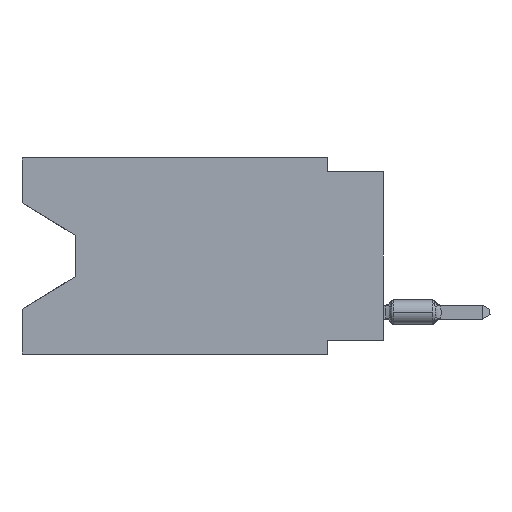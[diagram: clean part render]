
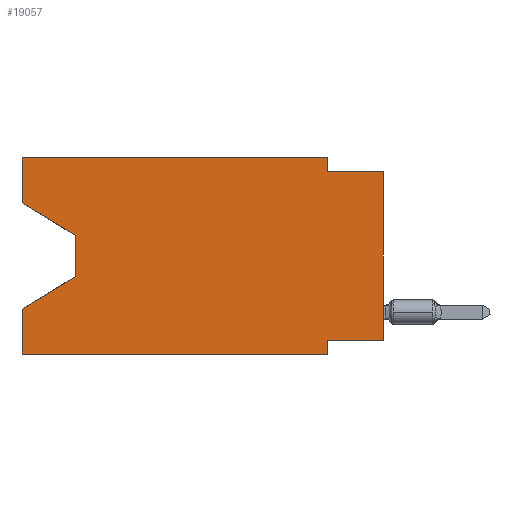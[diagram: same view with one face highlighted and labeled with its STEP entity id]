
A CAD part, left-side view. The second image highlights one B-rep face of the part: STEP entity #19057.
In plain terms, the highlighted planar face has unit normal (-1, 0, 0).
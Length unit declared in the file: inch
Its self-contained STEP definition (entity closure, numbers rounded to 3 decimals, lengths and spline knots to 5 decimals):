
#34 = VERTEX_POINT ( 'NONE', #14660 ) ;
#140 = VERTEX_POINT ( 'NONE', #9480 ) ;
#253 = EDGE_CURVE ( 'NONE', #2714, #13187, #6038, .T. ) ;
#280 = EDGE_CURVE ( 'NONE', #14166, #10763, #8495, .T. ) ;
#375 = ORIENTED_EDGE ( 'NONE', *, *, #20442, .F. ) ;
#603 = LINE ( 'NONE', #19292, #10857 ) ;
#1060 = DIRECTION ( 'NONE',  ( 0., 1., 0. ) ) ;
#1623 = ORIENTED_EDGE ( 'NONE', *, *, #253, .F. ) ;
#2714 = VERTEX_POINT ( 'NONE', #4708 ) ;
#2724 = EDGE_CURVE ( 'NONE', #13187, #140, #6681, .T. ) ;
#2912 = LINE ( 'NONE', #10428, #6878 ) ;
#2921 = VECTOR ( 'NONE', #8651, 39.37008 ) ;
#3528 = CARTESIAN_POINT ( 'NONE',  ( 0., 0.1, -0.325 ) ) ;
#3607 = EDGE_CURVE ( 'NONE', #140, #9707, #603, .T. ) ;
#4462 = DIRECTION ( 'NONE',  ( 0., 0., 1. ) ) ;
#4708 = CARTESIAN_POINT ( 'NONE',  ( 0., 0.645, 0. ) ) ;
#4752 = EDGE_CURVE ( 'NONE', #11798, #12851, #23490, .T. ) ;
#4802 = VERTEX_POINT ( 'NONE', #3528 ) ;
#5406 = ORIENTED_EDGE ( 'NONE', *, *, #13270, .T. ) ;
#5875 = ORIENTED_EDGE ( 'NONE', *, *, #4752, .F. ) ;
#6038 = LINE ( 'NONE', #23015, #8068 ) ;
#6166 = EDGE_CURVE ( 'NONE', #4802, #23695, #21912, .T. ) ;
#6455 = DIRECTION ( 'NONE',  ( 0., 0.855, -0.519 ) ) ;
#6636 = CARTESIAN_POINT ( 'NONE',  ( 0., 0.645, 0. ) ) ;
#6681 = LINE ( 'NONE', #8647, #7608 ) ;
#6878 = VECTOR ( 'NONE', #1060, 39.37008 ) ;
#7608 = VECTOR ( 'NONE', #23177, 39.37008 ) ;
#7696 = ORIENTED_EDGE ( 'NONE', *, *, #2724, .F. ) ;
#7800 = LINE ( 'NONE', #13824, #12699 ) ;
#8068 = VECTOR ( 'NONE', #13538, 39.37008 ) ;
#8118 = EDGE_CURVE ( 'NONE', #10763, #14246, #9164, .T. ) ;
#8310 = EDGE_CURVE ( 'NONE', #14246, #12851, #7800, .T. ) ;
#8495 = LINE ( 'NONE', #23128, #11324 ) ;
#8499 = ORIENTED_EDGE ( 'NONE', *, *, #8118, .T. ) ;
#8582 = CARTESIAN_POINT ( 'NONE',  ( 0., 0.55, -0.138 ) ) ;
#8647 = CARTESIAN_POINT ( 'NONE',  ( 0., 0.1, 0. ) ) ;
#8651 = DIRECTION ( 'NONE',  ( 0., 0., 1. ) ) ;
#8866 = CARTESIAN_POINT ( 'NONE',  ( 0., 0.1, -0.35 ) ) ;
#9164 = LINE ( 'NONE', #18997, #23437 ) ;
#9313 = PLANE ( 'NONE',  #19392 ) ;
#9387 = DIRECTION ( 'NONE',  ( 0., -1., 0. ) ) ;
#9480 = CARTESIAN_POINT ( 'NONE',  ( 0., 0.1, -0.025 ) ) ;
#9639 = LINE ( 'NONE', #19100, #23244 ) ;
#9693 = CARTESIAN_POINT ( 'NONE',  ( 0., 0.645, 0. ) ) ;
#9707 = VERTEX_POINT ( 'NONE', #18649 ) ;
#10134 = LINE ( 'NONE', #19473, #20805 ) ;
#10428 = CARTESIAN_POINT ( 'NONE',  ( 0., 0., -0.325 ) ) ;
#10763 = VERTEX_POINT ( 'NONE', #8582 ) ;
#10857 = VECTOR ( 'NONE', #21142, 39.37008 ) ;
#11324 = VECTOR ( 'NONE', #17594, 39.37008 ) ;
#11798 = VERTEX_POINT ( 'NONE', #19199 ) ;
#12699 = VECTOR ( 'NONE', #6455, 39.37008 ) ;
#12851 = VERTEX_POINT ( 'NONE', #14942 ) ;
#12917 = VECTOR ( 'NONE', #23121, 39.37008 ) ;
#13187 = VERTEX_POINT ( 'NONE', #22071 ) ;
#13270 = EDGE_CURVE ( 'NONE', #11798, #23695, #9639, .T. ) ;
#13538 = DIRECTION ( 'NONE',  ( 0., -1., 0. ) ) ;
#13815 = ORIENTED_EDGE ( 'NONE', *, *, #6166, .F. ) ;
#13824 = CARTESIAN_POINT ( 'NONE',  ( 0., 0.55, -0.212 ) ) ;
#14166 = VERTEX_POINT ( 'NONE', #22589 ) ;
#14246 = VERTEX_POINT ( 'NONE', #22819 ) ;
#14518 = DIRECTION ( 'NONE',  ( 0., 0., -1. ) ) ;
#14660 = CARTESIAN_POINT ( 'NONE',  ( 0., 0., -0.325 ) ) ;
#14942 = CARTESIAN_POINT ( 'NONE',  ( 0., 0.645, -0.26975 ) ) ;
#14963 = EDGE_LOOP ( 'NONE', ( #19547, #8499, #18477, #5875, #5406, #13815, #375, #15110, #23744, #7696, #1623, #16236 ) ) ;
#15110 = ORIENTED_EDGE ( 'NONE', *, *, #23382, .T. ) ;
#15488 = CARTESIAN_POINT ( 'NONE',  ( 0., 0.1, -0.35 ) ) ;
#16236 = ORIENTED_EDGE ( 'NONE', *, *, #19839, .F. ) ;
#16783 = DIRECTION ( 'NONE',  ( 0., 0., -1. ) ) ;
#17065 = DIRECTION ( 'NONE',  ( 1., 0., 0. ) ) ;
#17181 = DIRECTION ( 'NONE',  ( 0., 0., -1. ) ) ;
#17594 = DIRECTION ( 'NONE',  ( 0., -0.855, -0.519 ) ) ;
#18477 = ORIENTED_EDGE ( 'NONE', *, *, #8310, .T. ) ;
#18649 = CARTESIAN_POINT ( 'NONE',  ( 0., 0., -0.025 ) ) ;
#18787 = FACE_OUTER_BOUND ( 'NONE', #14963, .T. ) ;
#18997 = CARTESIAN_POINT ( 'NONE',  ( 0., 0.55, -0.138 ) ) ;
#19057 = ADVANCED_FACE ( 'NONE', ( #18787 ), #9313, .F. ) ;
#19100 = CARTESIAN_POINT ( 'NONE',  ( 0., 0.645, -0.35 ) ) ;
#19199 = CARTESIAN_POINT ( 'NONE',  ( 0., 0.645, -0.35 ) ) ;
#19292 = CARTESIAN_POINT ( 'NONE',  ( 0., 0., -0.025 ) ) ;
#19392 = AXIS2_PLACEMENT_3D ( 'NONE', #9693, #17065, #17181 ) ;
#19473 = CARTESIAN_POINT ( 'NONE',  ( 0., 0., 0. ) ) ;
#19547 = ORIENTED_EDGE ( 'NONE', *, *, #280, .T. ) ;
#19839 = EDGE_CURVE ( 'NONE', #14166, #2714, #19855, .T. ) ;
#19855 = LINE ( 'NONE', #19974, #2921 ) ;
#19974 = CARTESIAN_POINT ( 'NONE',  ( 0., 0.645, 0. ) ) ;
#20442 = EDGE_CURVE ( 'NONE', #34, #4802, #2912, .T. ) ;
#20805 = VECTOR ( 'NONE', #4462, 39.37008 ) ;
#21142 = DIRECTION ( 'NONE',  ( 0., -1., 0. ) ) ;
#21813 = VECTOR ( 'NONE', #14518, 39.37008 ) ;
#21912 = LINE ( 'NONE', #8866, #21813 ) ;
#22071 = CARTESIAN_POINT ( 'NONE',  ( 0., 0.1, 0. ) ) ;
#22589 = CARTESIAN_POINT ( 'NONE',  ( 0., 0.645, -0.08025 ) ) ;
#22819 = CARTESIAN_POINT ( 'NONE',  ( 0., 0.55, -0.212 ) ) ;
#23015 = CARTESIAN_POINT ( 'NONE',  ( 0., 0.645, 0. ) ) ;
#23121 = DIRECTION ( 'NONE',  ( 0., 0., 1. ) ) ;
#23128 = CARTESIAN_POINT ( 'NONE',  ( 0., 0.645, -0.08025 ) ) ;
#23177 = DIRECTION ( 'NONE',  ( 0., 0., -1. ) ) ;
#23244 = VECTOR ( 'NONE', #9387, 39.37008 ) ;
#23382 = EDGE_CURVE ( 'NONE', #34, #9707, #10134, .T. ) ;
#23437 = VECTOR ( 'NONE', #16783, 39.37008 ) ;
#23490 = LINE ( 'NONE', #6636, #12917 ) ;
#23695 = VERTEX_POINT ( 'NONE', #15488 ) ;
#23744 = ORIENTED_EDGE ( 'NONE', *, *, #3607, .F. ) ;
